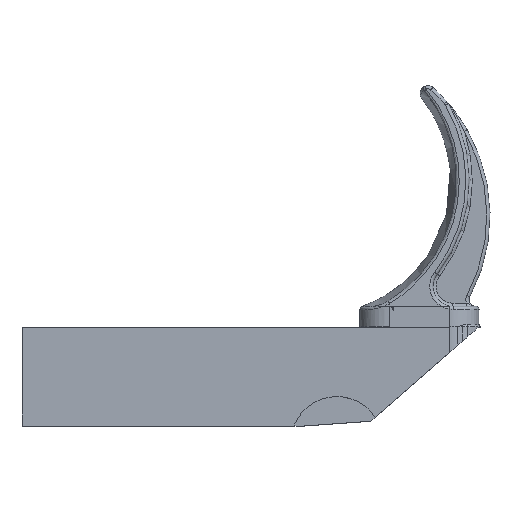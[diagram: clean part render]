
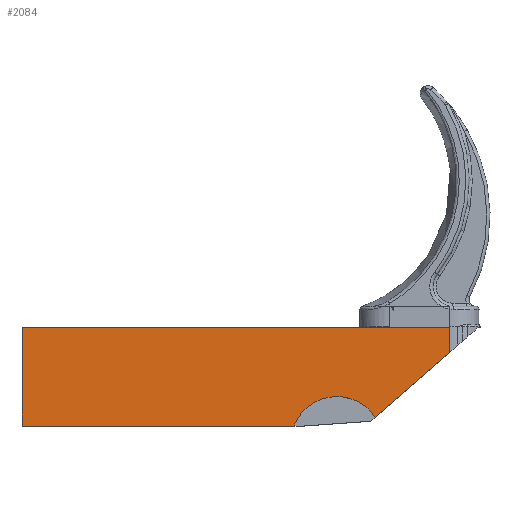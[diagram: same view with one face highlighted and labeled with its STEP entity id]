
A CAD part, top view. The second image highlights one B-rep face of the part: STEP entity #2084.
In plain terms, the highlighted planar face has unit normal (0, 0, 1).
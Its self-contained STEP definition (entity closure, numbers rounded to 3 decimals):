
#42=PLANE('',#2250);
#167=FACE_OUTER_BOUND('',#294,.T.);
#294=EDGE_LOOP('',(#1612,#1613,#1614,#1615,#1616,#1617,#1618,#1619));
#402=LINE('',#10771,#523);
#417=LINE('',#10808,#538);
#430=LINE('',#10846,#551);
#455=LINE('',#10975,#576);
#456=LINE('',#10979,#577);
#457=LINE('',#10980,#578);
#458=LINE('',#10981,#579);
#523=VECTOR('',#2488,10.);
#538=VECTOR('',#2519,10.);
#551=VECTOR('',#2564,10.);
#576=VECTOR('',#2609,10.);
#577=VECTOR('',#2612,10.);
#578=VECTOR('',#2613,10.);
#579=VECTOR('',#2614,10.);
#740=CIRCLE('',#2251,5.718);
#884=VERTEX_POINT('',#10768);
#885=VERTEX_POINT('',#10770);
#899=VERTEX_POINT('',#10806);
#907=VERTEX_POINT('',#10843);
#908=VERTEX_POINT('',#10845);
#926=VERTEX_POINT('',#10974);
#927=VERTEX_POINT('',#10976);
#928=VERTEX_POINT('',#10978);
#1108=EDGE_CURVE('',#885,#884,#402,.T.);
#1128=EDGE_CURVE('',#884,#899,#417,.T.);
#1146=EDGE_CURVE('',#908,#907,#430,.T.);
#1181=EDGE_CURVE('',#899,#926,#455,.T.);
#1182=EDGE_CURVE('',#926,#927,#740,.T.);
#1183=EDGE_CURVE('',#927,#928,#456,.T.);
#1184=EDGE_CURVE('',#928,#908,#457,.T.);
#1185=EDGE_CURVE('',#907,#885,#458,.T.);
#1612=ORIENTED_EDGE('',*,*,#1181,.T.);
#1613=ORIENTED_EDGE('',*,*,#1182,.T.);
#1614=ORIENTED_EDGE('',*,*,#1183,.T.);
#1615=ORIENTED_EDGE('',*,*,#1184,.T.);
#1616=ORIENTED_EDGE('',*,*,#1146,.T.);
#1617=ORIENTED_EDGE('',*,*,#1185,.T.);
#1618=ORIENTED_EDGE('',*,*,#1108,.T.);
#1619=ORIENTED_EDGE('',*,*,#1128,.T.);
#2084=ADVANCED_FACE('',(#167),#42,.T.);
#2250=AXIS2_PLACEMENT_3D('',#10973,#2607,#2608);
#2251=AXIS2_PLACEMENT_3D('',#10977,#2610,#2611);
#2488=DIRECTION('',(-1.,0.,0.));
#2519=DIRECTION('',(0.,-1.,0.));
#2564=DIRECTION('',(-1.,0.,0.));
#2607=DIRECTION('center_axis',(0.,0.,1.));
#2608=DIRECTION('ref_axis',(1.,0.,0.));
#2609=DIRECTION('',(1.,0.,0.));
#2610=DIRECTION('center_axis',(0.,0.,-1.));
#2611=DIRECTION('ref_axis',(-0.997,-0.071,0.));
#2612=DIRECTION('',(0.754,0.657,0.));
#2613=DIRECTION('',(0.,1.,0.));
#2614=DIRECTION('',(0.,-1.,0.));
#10768=CARTESIAN_POINT('',(30.4,-8.476,4.683));
#10770=CARTESIAN_POINT('',(30.414,-8.476,4.683));
#10771=CARTESIAN_POINT('',(30.414,-8.476,4.683));
#10806=CARTESIAN_POINT('',(30.4,-12.259,4.683));
#10808=CARTESIAN_POINT('',(30.4,-8.476,4.683));
#10843=CARTESIAN_POINT('',(30.414,0.,4.683));
#10845=CARTESIAN_POINT('',(83.427,0.,4.683));
#10846=CARTESIAN_POINT('',(76.,0.,4.683));
#10973=CARTESIAN_POINT('Origin',(56.867,-5.476,4.683));
#10974=CARTESIAN_POINT('',(64.125,-12.259,4.683));
#10975=CARTESIAN_POINT('',(30.4,-12.259,4.683));
#10976=CARTESIAN_POINT('',(74.23,-11.133,4.683));
#10977=CARTESIAN_POINT('Origin',(69.467,-14.298,4.683));
#10978=CARTESIAN_POINT('',(83.427,-3.115,4.683));
#10979=CARTESIAN_POINT('',(73.648,-11.641,4.683));
#10980=CARTESIAN_POINT('',(83.427,-3.115,4.683));
#10981=CARTESIAN_POINT('',(30.414,0.,4.683));
